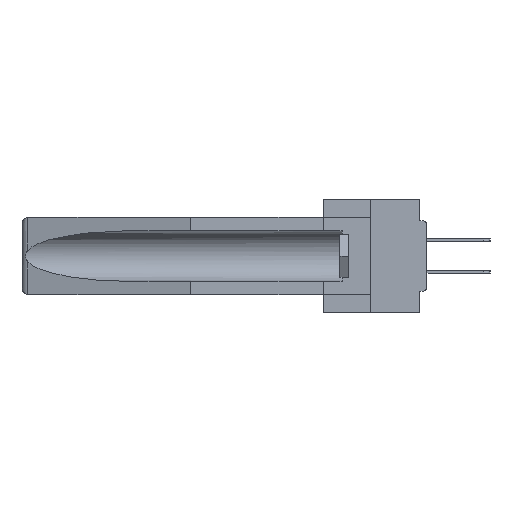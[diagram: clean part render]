
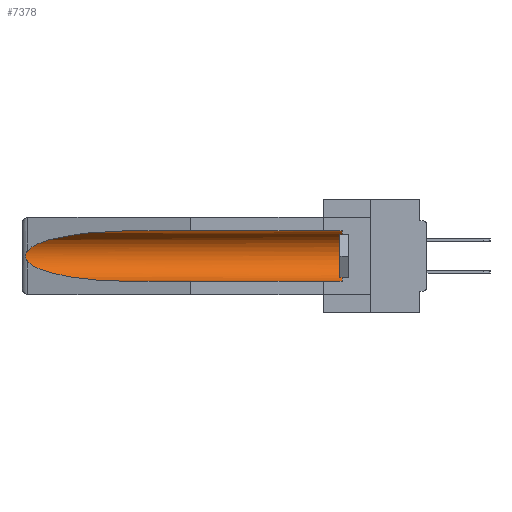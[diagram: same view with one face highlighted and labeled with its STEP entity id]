
A CAD part, left-side view. The second image highlights one B-rep face of the part: STEP entity #7378.
In plain terms, the highlighted cylindrical face has radius 2.857 mm (diameter 5.715 mm), a partial arc.
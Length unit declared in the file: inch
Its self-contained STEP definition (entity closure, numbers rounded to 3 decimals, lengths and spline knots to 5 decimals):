
#426 = CARTESIAN_POINT ( 'NONE',  ( 0.25451, 1.48313, -0.24835 ) ) ;
#512 = ORIENTED_EDGE ( 'NONE', *, *, #31870, .T. ) ;
#1184 = ORIENTED_EDGE ( 'NONE', *, *, #31418, .F. ) ;
#1691 = CARTESIAN_POINT ( 'NONE',  ( 0.155, 1.07973, -0.284 ) ) ;
#2995 = VERTEX_POINT ( 'NONE', #8947 ) ;
#3505 = CARTESIAN_POINT ( 'NONE',  ( 0.26537, 1.52718, -0.14972 ) ) ;
#4197 = CYLINDRICAL_SURFACE ( 'NONE', #13489, 0.1125 ) ;
#4300 = CARTESIAN_POINT ( 'NONE',  ( 0.155, 1.07973, -0.059 ) ) ;
#4967 = CIRCLE ( 'NONE', #25879, 0.1125 ) ;
#7378 = ADVANCED_FACE ( 'NONE', ( #14230 ), #4197, .F. ) ;
#7482 = CARTESIAN_POINT ( 'NONE',  ( 0.21114, 1.30732, -0.059 ) ) ;
#7698 =( BOUNDED_CURVE ( )  B_SPLINE_CURVE ( 3, ( #4300, #7482, #25603, #9689 ),
 .UNSPECIFIED., .F., .F. ) 
 B_SPLINE_CURVE_WITH_KNOTS ( ( 4, 4 ),
 ( 4.71239, 6.08839 ),
 .UNSPECIFIED. ) 
 CURVE ( )  GEOMETRIC_REPRESENTATION_ITEM ( )  RATIONAL_B_SPLINE_CURVE ( ( 1., 0.848, 0.848, 1. ) ) 
 REPRESENTATION_ITEM ( '' )  );
#8419 = ORIENTED_EDGE ( 'NONE', *, *, #14302, .T. ) ;
#8634 = VERTEX_POINT ( 'NONE', #1691 ) ;
#8947 = CARTESIAN_POINT ( 'NONE',  ( 0.26537, 1.52718, -0.14972 ) ) ;
#9689 = CARTESIAN_POINT ( 'NONE',  ( 0.26537, 1.52718, -0.14972 ) ) ;
#10875 = EDGE_CURVE ( 'NONE', #23768, #2995, #7698, .T. ) ;
#10907 = ORIENTED_EDGE ( 'NONE', *, *, #20221, .T. ) ;
#11306 = B_SPLINE_CURVE_WITH_KNOTS ( 'NONE', 3,
 ( #3505, #11350, #27469, #24706, #11456, #16958, #14039, #30032, #14390, #16716 ),
 .UNSPECIFIED., .F., .F.,
 ( 4, 2, 2, 2, 4 ),
 ( 0., 0.00029, 0.00058, 0.00087, 0.00117 ),
 .UNSPECIFIED. ) ;
#11350 = CARTESIAN_POINT ( 'NONE',  ( 0.26597, 1.52961, -0.15275 ) ) ;
#11456 = CARTESIAN_POINT ( 'NONE',  ( 0.2675, 1.53308, -0.16763 ) ) ;
#12597 = DIRECTION ( 'NONE',  ( 0., 1., 0. ) ) ;
#12833 = DIRECTION ( 'NONE',  ( 0., 0., 1. ) ) ;
#13489 = AXIS2_PLACEMENT_3D ( 'NONE', #15288, #12597, #12833 ) ;
#14039 = CARTESIAN_POINT ( 'NONE',  ( 0.2673, 1.53269, -0.17917 ) ) ;
#14230 = FACE_OUTER_BOUND ( 'NONE', #31823, .T. ) ;
#14302 = EDGE_CURVE ( 'NONE', #22363, #8634, #33441, .T. ) ;
#14390 = CARTESIAN_POINT ( 'NONE',  ( 0.26597, 1.5296, -0.19026 ) ) ;
#15288 = CARTESIAN_POINT ( 'NONE',  ( 0.155, -0.30754, -0.1715 ) ) ;
#16716 = CARTESIAN_POINT ( 'NONE',  ( 0.26537, 1.52718, -0.19328 ) ) ;
#16958 = CARTESIAN_POINT ( 'NONE',  ( 0.2675, 1.53308, -0.17534 ) ) ;
#18012 = VECTOR ( 'NONE', #23306, 39.37008 ) ;
#18619 = CARTESIAN_POINT ( 'NONE',  ( 0.155, 0.126, -0.1715 ) ) ;
#18925 = CARTESIAN_POINT ( 'NONE',  ( 0.155, 0.126, -0.059 ) ) ;
#20221 = EDGE_CURVE ( 'NONE', #31480, #23768, #32005, .T. ) ;
#20387 = EDGE_CURVE ( 'NONE', #20868, #31480, #4967, .T. ) ;
#20868 = VERTEX_POINT ( 'NONE', #33618 ) ;
#21264 = DIRECTION ( 'NONE',  ( 0., -1., 0. ) ) ;
#21378 = CARTESIAN_POINT ( 'NONE',  ( 0.155, 1.07973, -0.059 ) ) ;
#22096 = CARTESIAN_POINT ( 'NONE',  ( 0.21114, 1.30732, -0.284 ) ) ;
#22363 = VERTEX_POINT ( 'NONE', #25714 ) ;
#22987 = DIRECTION ( 'NONE',  ( 0., 1., 0. ) ) ;
#23306 = DIRECTION ( 'NONE',  ( 0., 1., 0. ) ) ;
#23613 = ORIENTED_EDGE ( 'NONE', *, *, #20387, .T. ) ;
#23768 = VERTEX_POINT ( 'NONE', #21378 ) ;
#23929 = DIRECTION ( 'NONE',  ( 0., 0., 1. ) ) ;
#24706 = CARTESIAN_POINT ( 'NONE',  ( 0.2673, 1.5327, -0.16383 ) ) ;
#25019 = LINE ( 'NONE', #33270, #18012 ) ;
#25205 = ORIENTED_EDGE ( 'NONE', *, *, #10875, .T. ) ;
#25603 = CARTESIAN_POINT ( 'NONE',  ( 0.25451, 1.48313, -0.09465 ) ) ;
#25714 = CARTESIAN_POINT ( 'NONE',  ( 0.26537, 1.52718, -0.19328 ) ) ;
#25879 = AXIS2_PLACEMENT_3D ( 'NONE', #18619, #21264, #23929 ) ;
#27469 = CARTESIAN_POINT ( 'NONE',  ( 0.26654, 1.53092, -0.15636 ) ) ;
#29645 = CARTESIAN_POINT ( 'NONE',  ( 0.26537, 1.52718, -0.19328 ) ) ;
#30032 = CARTESIAN_POINT ( 'NONE',  ( 0.26655, 1.53094, -0.18657 ) ) ;
#31418 = EDGE_CURVE ( 'NONE', #20868, #8634, #25019, .T. ) ;
#31480 = VERTEX_POINT ( 'NONE', #18925 ) ;
#31823 = EDGE_LOOP ( 'NONE', ( #25205, #512, #8419, #1184, #23613, #10907 ) ) ;
#31870 = EDGE_CURVE ( 'NONE', #2995, #22363, #11306, .T. ) ;
#32005 = LINE ( 'NONE', #33667, #32806 ) ;
#32302 = CARTESIAN_POINT ( 'NONE',  ( 0.155, 1.07973, -0.284 ) ) ;
#32806 = VECTOR ( 'NONE', #22987, 39.37008 ) ;
#33270 = CARTESIAN_POINT ( 'NONE',  ( 0.155, -0.30754, -0.284 ) ) ;
#33441 =( BOUNDED_CURVE ( )  B_SPLINE_CURVE ( 3, ( #29645, #426, #22096, #32302 ),
 .UNSPECIFIED., .F., .F. ) 
 B_SPLINE_CURVE_WITH_KNOTS ( ( 4, 4 ),
 ( 0.1948, 1.5708 ),
 .UNSPECIFIED. ) 
 CURVE ( )  GEOMETRIC_REPRESENTATION_ITEM ( )  RATIONAL_B_SPLINE_CURVE ( ( 1., 0.848, 0.848, 1. ) ) 
 REPRESENTATION_ITEM ( '' )  );
#33618 = CARTESIAN_POINT ( 'NONE',  ( 0.155, 0.126, -0.284 ) ) ;
#33667 = CARTESIAN_POINT ( 'NONE',  ( 0.155, -0.30754, -0.059 ) ) ;
